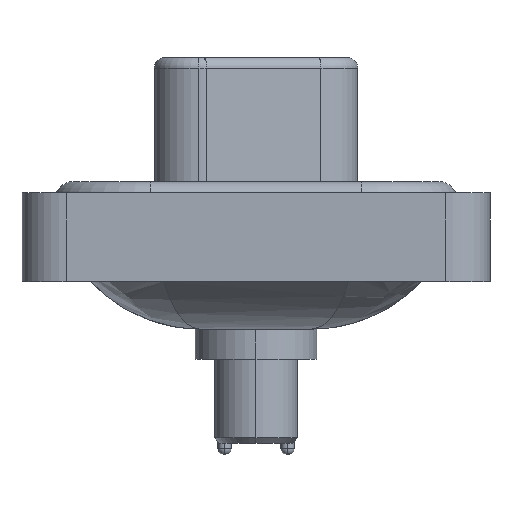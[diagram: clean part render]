
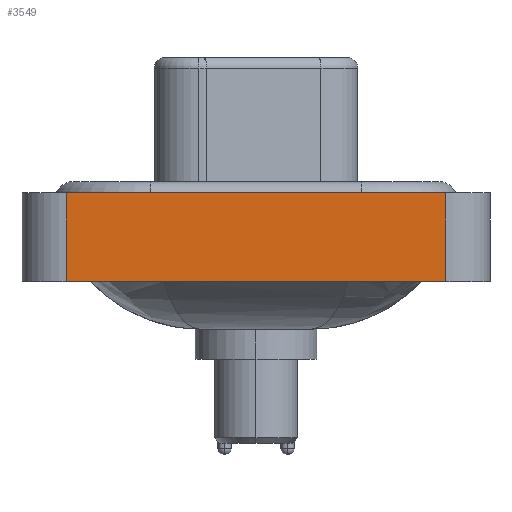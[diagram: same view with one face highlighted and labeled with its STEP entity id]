
A CAD part, left-side view. The second image highlights one B-rep face of the part: STEP entity #3549.
In plain terms, the highlighted planar face has unit normal (-1, 0, 0).
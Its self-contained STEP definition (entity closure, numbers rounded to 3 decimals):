
#91 = VECTOR ( 'NONE', #22116, 1000. ) ;
#507 = DIRECTION ( 'NONE',  ( 0., 0., 1. ) ) ;
#737 = FACE_OUTER_BOUND ( 'NONE', #3745, .T. ) ;
#949 = VECTOR ( 'NONE', #23182, 1000. ) ;
#2337 = CARTESIAN_POINT ( 'NONE',  ( -7.35, 8.55, 0.4 ) ) ;
#3549 = ADVANCED_FACE ( 'NONE', ( #737 ), #20148, .T. ) ;
#3745 = EDGE_LOOP ( 'NONE', ( #10918, #15486, #10278, #11633 ) ) ;
#6147 = CARTESIAN_POINT ( 'NONE',  ( -7.35, -8.55, -3.6 ) ) ;
#8804 = CARTESIAN_POINT ( 'NONE',  ( -7.35, -8.55, 0.4 ) ) ;
#9265 = EDGE_CURVE ( 'NONE', #15079, #13075, #20546, .T. ) ;
#10278 = ORIENTED_EDGE ( 'NONE', *, *, #9265, .F. ) ;
#10918 = ORIENTED_EDGE ( 'NONE', *, *, #22480, .T. ) ;
#11633 = ORIENTED_EDGE ( 'NONE', *, *, #11995, .T. ) ;
#11995 = EDGE_CURVE ( 'NONE', #15079, #22935, #16707, .T. ) ;
#13075 = VERTEX_POINT ( 'NONE', #2337 ) ;
#13105 = CARTESIAN_POINT ( 'NONE',  ( -7.35, -8.55, -3.6 ) ) ;
#13485 = VECTOR ( 'NONE', #20523, 1000. ) ;
#13493 = CARTESIAN_POINT ( 'NONE',  ( -7.35, -8.55, -3.6 ) ) ;
#13653 = VECTOR ( 'NONE', #18655, 1000. ) ;
#15079 = VERTEX_POINT ( 'NONE', #15488 ) ;
#15486 = ORIENTED_EDGE ( 'NONE', *, *, #18499, .F. ) ;
#15488 = CARTESIAN_POINT ( 'NONE',  ( -7.35, 8.55, -3.6 ) ) ;
#15870 = CARTESIAN_POINT ( 'NONE',  ( -7.35, -8.55, 0.4 ) ) ;
#16631 = DIRECTION ( 'NONE',  ( -1., 0., 0. ) ) ;
#16707 = LINE ( 'NONE', #22236, #91 ) ;
#17229 = LINE ( 'NONE', #13493, #13485 ) ;
#18499 = EDGE_CURVE ( 'NONE', #13075, #23081, #19416, .T. ) ;
#18655 = DIRECTION ( 'NONE',  ( 0., 0., 1. ) ) ;
#19416 = LINE ( 'NONE', #8804, #949 ) ;
#20148 = PLANE ( 'NONE',  #23202 ) ;
#20523 = DIRECTION ( 'NONE',  ( 0., 0., 1. ) ) ;
#20546 = LINE ( 'NONE', #22662, #13653 ) ;
#22116 = DIRECTION ( 'NONE',  ( 0., -1., 0. ) ) ;
#22236 = CARTESIAN_POINT ( 'NONE',  ( -7.35, -8.55, -3.6 ) ) ;
#22480 = EDGE_CURVE ( 'NONE', #22935, #23081, #17229, .T. ) ;
#22662 = CARTESIAN_POINT ( 'NONE',  ( -7.35, 8.55, -3.6 ) ) ;
#22935 = VERTEX_POINT ( 'NONE', #13105 ) ;
#23081 = VERTEX_POINT ( 'NONE', #15870 ) ;
#23182 = DIRECTION ( 'NONE',  ( 0., -1., 0. ) ) ;
#23202 = AXIS2_PLACEMENT_3D ( 'NONE', #6147, #16631, #507 ) ;
